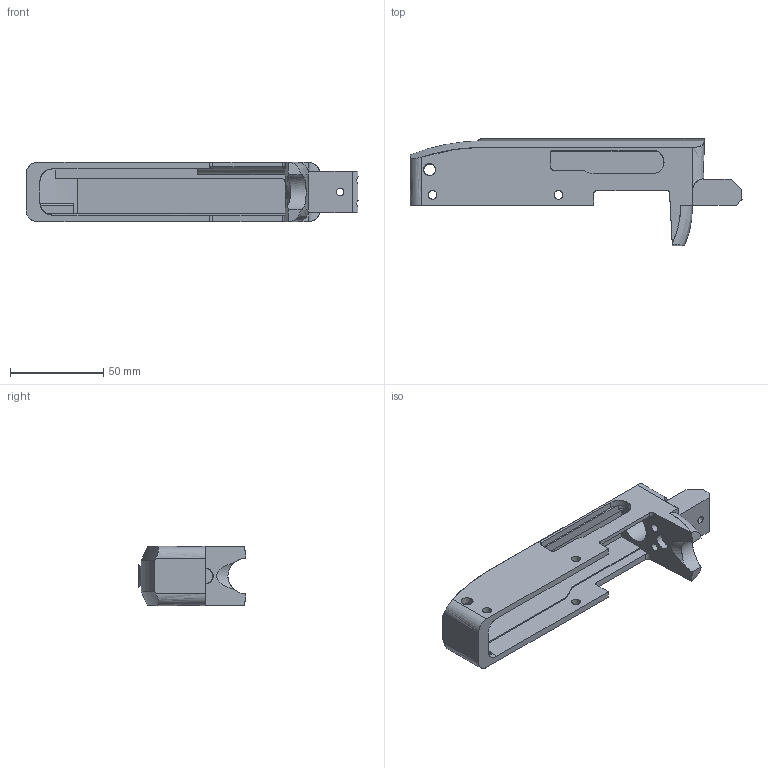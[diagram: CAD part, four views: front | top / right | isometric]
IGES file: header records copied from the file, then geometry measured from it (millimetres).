
Global section: file name: 10-22 Receiver Model.igs; native system: Virtual 7.7.6 NLO; preprocessor: Exchange 1.0; author: Tim Winkfein; organization: dumpsterCNC; date: 061101.042517; units: inch
Bounding box: 177.8 x 57.66 x 31.75 mm (x, y, z)
Surface area: 34160 mm2 (no closed solid volume)
Topology: 0 solids, 0 shells, 111 faces, 1607 edges, 1599 vertices
Faces by surface type: bspline 111
